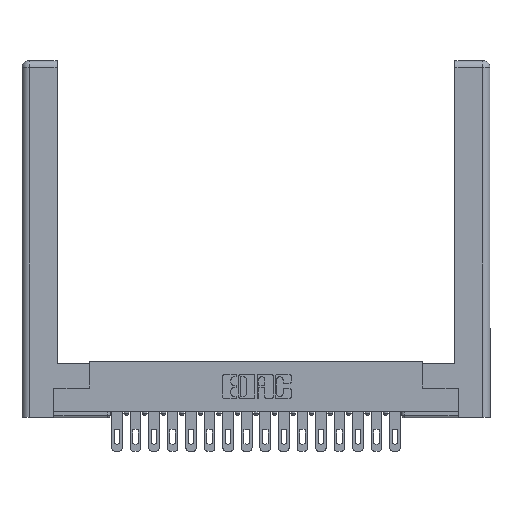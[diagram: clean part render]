
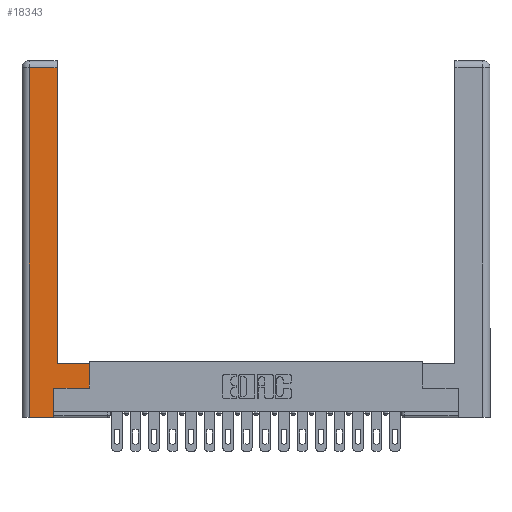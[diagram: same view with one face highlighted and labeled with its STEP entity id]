
A CAD part, top view. The second image highlights one B-rep face of the part: STEP entity #18343.
In plain terms, the highlighted planar face has unit normal (0, 0, 1).
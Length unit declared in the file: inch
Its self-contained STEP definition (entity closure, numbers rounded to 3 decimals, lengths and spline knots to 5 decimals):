
#60 = DIRECTION ( 'NONE',  ( -1., 0., 0. ) ) ;
#326 = LINE ( 'NONE', #18706, #15708 ) ;
#461 = VECTOR ( 'NONE', #14920, 39.37008 ) ;
#1560 = DIRECTION ( 'NONE',  ( 1., 0., 0. ) ) ;
#1672 = CARTESIAN_POINT ( 'NONE',  ( 0.295, 2.94, 0. ) ) ;
#1820 = VERTEX_POINT ( 'NONE', #9971 ) ;
#1959 = ORIENTED_EDGE ( 'NONE', *, *, #14063, .T. ) ;
#2634 = DIRECTION ( 'NONE',  ( 0., 0., -1. ) ) ;
#3200 = VECTOR ( 'NONE', #9270, 39.37008 ) ;
#3497 = AXIS2_PLACEMENT_3D ( 'NONE', #5585, #2634, #11763 ) ;
#3906 = CARTESIAN_POINT ( 'NONE',  ( 0.0615, 0., 0. ) ) ;
#4161 = CARTESIAN_POINT ( 'NONE',  ( 0.295, 3., 0. ) ) ;
#4189 = CARTESIAN_POINT ( 'NONE',  ( 0.0615, 0., 0. ) ) ;
#4381 = CARTESIAN_POINT ( 'NONE',  ( 0.265, 0., 0. ) ) ;
#4579 = EDGE_CURVE ( 'NONE', #6929, #16806, #12154, .T. ) ;
#5190 = CARTESIAN_POINT ( 'NONE',  ( 0.565, 0.245, 0. ) ) ;
#5273 = ORIENTED_EDGE ( 'NONE', *, *, #4579, .T. ) ;
#5291 = ORIENTED_EDGE ( 'NONE', *, *, #14990, .T. ) ;
#5478 = EDGE_CURVE ( 'NONE', #16261, #9746, #7587, .T. ) ;
#5585 = CARTESIAN_POINT ( 'NONE',  ( 0., 0., 0. ) ) ;
#5995 = CARTESIAN_POINT ( 'NONE',  ( 0.565, 0.45, 0. ) ) ;
#6929 = VERTEX_POINT ( 'NONE', #5995 ) ;
#7120 = FACE_OUTER_BOUND ( 'NONE', #9111, .T. ) ;
#7587 = LINE ( 'NONE', #12326, #17911 ) ;
#7604 = DIRECTION ( 'NONE',  ( 0., 1., 0. ) ) ;
#9111 = EDGE_LOOP ( 'NONE', ( #5291, #20056, #13549, #12144, #1959, #11282, #12480, #5273 ) ) ;
#9270 = DIRECTION ( 'NONE',  ( 0., -1., 0. ) ) ;
#9746 = VERTEX_POINT ( 'NONE', #5190 ) ;
#9887 = DIRECTION ( 'NONE',  ( 0., 1., 0. ) ) ;
#9968 = LINE ( 'NONE', #4161, #461 ) ;
#9971 = CARTESIAN_POINT ( 'NONE',  ( 0.0615, 2.94, 0. ) ) ;
#10372 = EDGE_CURVE ( 'NONE', #17172, #1820, #10503, .T. ) ;
#10503 = LINE ( 'NONE', #15176, #19166 ) ;
#11282 = ORIENTED_EDGE ( 'NONE', *, *, #5478, .T. ) ;
#11763 = DIRECTION ( 'NONE',  ( -1., 0., 0. ) ) ;
#11821 = VECTOR ( 'NONE', #16239, 39.37008 ) ;
#11848 = LINE ( 'NONE', #15297, #14747 ) ;
#11873 = CARTESIAN_POINT ( 'NONE',  ( 0.265, 0., 0. ) ) ;
#11899 = LINE ( 'NONE', #4189, #3200 ) ;
#12144 = ORIENTED_EDGE ( 'NONE', *, *, #15016, .T. ) ;
#12154 = LINE ( 'NONE', #18538, #18397 ) ;
#12326 = CARTESIAN_POINT ( 'NONE',  ( 0.565, 0.245, 0. ) ) ;
#12480 = ORIENTED_EDGE ( 'NONE', *, *, #13028, .T. ) ;
#12861 = DIRECTION ( 'NONE',  ( -1., 0., 0. ) ) ;
#13028 = EDGE_CURVE ( 'NONE', #9746, #6929, #326, .T. ) ;
#13299 = PLANE ( 'NONE',  #3497 ) ;
#13549 = ORIENTED_EDGE ( 'NONE', *, *, #19312, .T. ) ;
#14063 = EDGE_CURVE ( 'NONE', #15178, #16261, #11848, .T. ) ;
#14747 = VECTOR ( 'NONE', #7604, 39.37008 ) ;
#14920 = DIRECTION ( 'NONE',  ( 0., 1., 0. ) ) ;
#14990 = EDGE_CURVE ( 'NONE', #16806, #17172, #9968, .T. ) ;
#15016 = EDGE_CURVE ( 'NONE', #17323, #15178, #17848, .T. ) ;
#15176 = CARTESIAN_POINT ( 'NONE',  ( 0.0615, 2.94, 0. ) ) ;
#15178 = VERTEX_POINT ( 'NONE', #4381 ) ;
#15297 = CARTESIAN_POINT ( 'NONE',  ( 0.265, 0.245, 0. ) ) ;
#15708 = VECTOR ( 'NONE', #9887, 39.37008 ) ;
#16139 = CARTESIAN_POINT ( 'NONE',  ( 0.295, 0.45, 0. ) ) ;
#16239 = DIRECTION ( 'NONE',  ( 1., 0., 0. ) ) ;
#16261 = VERTEX_POINT ( 'NONE', #19119 ) ;
#16806 = VERTEX_POINT ( 'NONE', #16139 ) ;
#17172 = VERTEX_POINT ( 'NONE', #1672 ) ;
#17323 = VERTEX_POINT ( 'NONE', #3906 ) ;
#17848 = LINE ( 'NONE', #11873, #11821 ) ;
#17911 = VECTOR ( 'NONE', #1560, 39.37008 ) ;
#18343 = ADVANCED_FACE ( 'NONE', ( #7120 ), #13299, .F. ) ;
#18397 = VECTOR ( 'NONE', #60, 39.37008 ) ;
#18538 = CARTESIAN_POINT ( 'NONE',  ( 0.295, 0.45, 0. ) ) ;
#18706 = CARTESIAN_POINT ( 'NONE',  ( 0.565, 0.45, 0. ) ) ;
#19119 = CARTESIAN_POINT ( 'NONE',  ( 0.265, 0.245, 0. ) ) ;
#19166 = VECTOR ( 'NONE', #12861, 39.37008 ) ;
#19312 = EDGE_CURVE ( 'NONE', #1820, #17323, #11899, .T. ) ;
#20056 = ORIENTED_EDGE ( 'NONE', *, *, #10372, .T. ) ;
